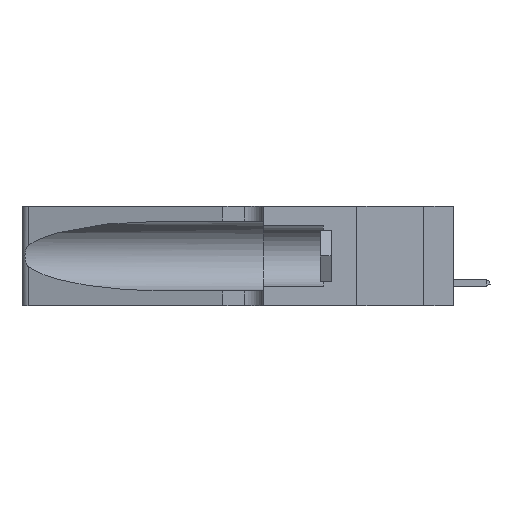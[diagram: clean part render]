
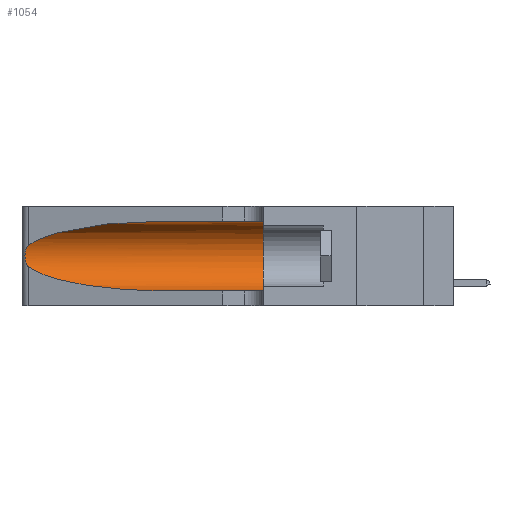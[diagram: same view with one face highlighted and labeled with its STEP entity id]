
A CAD part, left-side view. The second image highlights one B-rep face of the part: STEP entity #1054.
In plain terms, the highlighted cylindrical face has radius 3.308 mm (diameter 6.617 mm), a partial arc.
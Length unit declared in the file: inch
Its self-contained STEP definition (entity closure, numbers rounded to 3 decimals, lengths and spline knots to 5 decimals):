
#74 = ORIENTED_EDGE ( 'NONE', *, *, #16805, .F. ) ;
#197 = VERTEX_POINT ( 'NONE', #497 ) ;
#427 = CARTESIAN_POINT ( 'NONE',  ( 0.1305, 0.72297, 0.31525 ) ) ;
#497 = CARTESIAN_POINT ( 'NONE',  ( 0.1305, 0.72297, 0.31525 ) ) ;
#614 = CARTESIAN_POINT ( 'NONE',  ( 0.25487, 1.22718, 0.22369 ) ) ;
#639 = AXIS2_PLACEMENT_3D ( 'NONE', #3999, #11003, #16444 ) ;
#1054 = ADVANCED_FACE ( 'NONE', ( #14045 ), #2407, .F. ) ;
#1343 = VERTEX_POINT ( 'NONE', #614 ) ;
#1510 = CARTESIAN_POINT ( 'NONE',  ( 0.25487, 1.22718, 0.14631 ) ) ;
#2016 = VECTOR ( 'NONE', #13658, 39.37008 ) ;
#2313 = CARTESIAN_POINT ( 'NONE',  ( 0.25787, 1.23484, 0.2124 ) ) ;
#2407 = CYLINDRICAL_SURFACE ( 'NONE', #639, 0.13025 ) ;
#2548 = CARTESIAN_POINT ( 'NONE',  ( 0.25487, 1.22718, 0.14631 ) ) ;
#2901 = VERTEX_POINT ( 'NONE', #11249 ) ;
#3780 = B_SPLINE_CURVE_WITH_KNOTS ( 'NONE', 3,
 ( #16216, #17584, #7789, #2313, #9340, #13317, #3889, #9224, #8253, #17644, #8194, #9400, #16392, #2548 ),
 .UNSPECIFIED., .F., .F.,
 ( 4, 2, 2, 2, 2, 2, 4 ),
 ( 0., 0.00027, 0.00053, 0.00107, 0.0016, 0.00187, 0.00214 ),
 .UNSPECIFIED. ) ;
#3876 = EDGE_CURVE ( 'NONE', #4979, #2901, #10930, .T. ) ;
#3889 = CARTESIAN_POINT ( 'NONE',  ( 0.26075, 1.23896, 0.19203 ) ) ;
#3999 = CARTESIAN_POINT ( 'NONE',  ( 0.1305, 1.61858, 0.185 ) ) ;
#4387 = CIRCLE ( 'NONE', #9984, 0.13025 ) ;
#4979 = VERTEX_POINT ( 'NONE', #14927 ) ;
#5138 = DIRECTION ( 'NONE',  ( 0., 1., 0. ) ) ;
#5462 = ORIENTED_EDGE ( 'NONE', *, *, #14067, .F. ) ;
#5634 = CARTESIAN_POINT ( 'NONE',  ( 0.1305, 0.72297, 0.05475 ) ) ;
#6020 = ORIENTED_EDGE ( 'NONE', *, *, #17604, .T. ) ;
#6973 = LINE ( 'NONE', #6981, #2016 ) ;
#6981 = CARTESIAN_POINT ( 'NONE',  ( 0.1305, 1.61858, 0.31525 ) ) ;
#7063 = CARTESIAN_POINT ( 'NONE',  ( 0.1305, 1.61858, 0.05475 ) ) ;
#7192 = CARTESIAN_POINT ( 'NONE',  ( 0.25487, 1.22718, 0.22369 ) ) ;
#7325 = EDGE_CURVE ( 'NONE', #1343, #17006, #3780, .T. ) ;
#7789 = CARTESIAN_POINT ( 'NONE',  ( 0.25639, 1.23184, 0.21858 ) ) ;
#8151 = ORIENTED_EDGE ( 'NONE', *, *, #7325, .T. ) ;
#8194 = CARTESIAN_POINT ( 'NONE',  ( 0.25789, 1.23486, 0.15765 ) ) ;
#8253 = CARTESIAN_POINT ( 'NONE',  ( 0.26017, 1.23833, 0.17102 ) ) ;
#8424 = DIRECTION ( 'NONE',  ( 0., -1., 0. ) ) ;
#8612 = CARTESIAN_POINT ( 'NONE',  ( 0.18966, 0.96281, 0.31525 ) ) ;
#9224 = CARTESIAN_POINT ( 'NONE',  ( 0.26075, 1.23896, 0.178 ) ) ;
#9231 = VECTOR ( 'NONE', #8424, 39.37008 ) ;
#9340 = CARTESIAN_POINT ( 'NONE',  ( 0.25854, 1.2359, 0.20912 ) ) ;
#9400 = CARTESIAN_POINT ( 'NONE',  ( 0.25639, 1.23186, 0.15144 ) ) ;
#9636 = EDGE_CURVE ( 'NONE', #17006, #4979, #13362, .T. ) ;
#9984 = AXIS2_PLACEMENT_3D ( 'NONE', #13387, #5138, #15196 ) ;
#10185 = CARTESIAN_POINT ( 'NONE',  ( 0.25487, 1.22718, 0.14631 ) ) ;
#10930 = LINE ( 'NONE', #7063, #9231 ) ;
#11003 = DIRECTION ( 'NONE',  ( 0., -1., 0. ) ) ;
#11182 = CARTESIAN_POINT ( 'NONE',  ( 0.2373, 1.15595, 0.08982 ) ) ;
#11249 = CARTESIAN_POINT ( 'NONE',  ( 0.1305, 0.35, 0.05475 ) ) ;
#13317 = CARTESIAN_POINT ( 'NONE',  ( 0.26018, 1.23835, 0.19895 ) ) ;
#13362 =( BOUNDED_CURVE ( )  B_SPLINE_CURVE ( 3, ( #1510, #11182, #13901, #5634 ),
 .UNSPECIFIED., .F., .T. ) 
 B_SPLINE_CURVE_WITH_KNOTS ( ( 4, 4 ),
 ( 3.44316, 4.71239 ),
 .UNSPECIFIED. ) 
 CURVE ( )  GEOMETRIC_REPRESENTATION_ITEM ( )  RATIONAL_B_SPLINE_CURVE ( ( 1., 0.87, 0.87, 1. ) ) 
 REPRESENTATION_ITEM ( '' )  );
#13387 = CARTESIAN_POINT ( 'NONE',  ( 0.1305, 0.35, 0.185 ) ) ;
#13569 = VERTEX_POINT ( 'NONE', #14386 ) ;
#13658 = DIRECTION ( 'NONE',  ( 0., -1., 0. ) ) ;
#13901 = CARTESIAN_POINT ( 'NONE',  ( 0.18966, 0.96281, 0.05475 ) ) ;
#14045 = FACE_OUTER_BOUND ( 'NONE', #16187, .T. ) ;
#14067 = EDGE_CURVE ( 'NONE', #197, #13569, #6973, .T. ) ;
#14386 = CARTESIAN_POINT ( 'NONE',  ( 0.1305, 0.35, 0.31525 ) ) ;
#14625 = ORIENTED_EDGE ( 'NONE', *, *, #3876, .T. ) ;
#14927 = CARTESIAN_POINT ( 'NONE',  ( 0.1305, 0.72297, 0.05475 ) ) ;
#15196 = DIRECTION ( 'NONE',  ( 0., 0., 1. ) ) ;
#15252 =( BOUNDED_CURVE ( )  B_SPLINE_CURVE ( 3, ( #427, #8612, #15593, #7192 ),
 .UNSPECIFIED., .F., .F. ) 
 B_SPLINE_CURVE_WITH_KNOTS ( ( 4, 4 ),
 ( 1.5708, 2.84003 ),
 .UNSPECIFIED. ) 
 CURVE ( )  GEOMETRIC_REPRESENTATION_ITEM ( )  RATIONAL_B_SPLINE_CURVE ( ( 1., 0.87, 0.87, 1. ) ) 
 REPRESENTATION_ITEM ( '' )  );
#15593 = CARTESIAN_POINT ( 'NONE',  ( 0.2373, 1.15595, 0.28018 ) ) ;
#16187 = EDGE_LOOP ( 'NONE', ( #6020, #8151, #17337, #14625, #74, #5462 ) ) ;
#16216 = CARTESIAN_POINT ( 'NONE',  ( 0.25487, 1.22718, 0.22369 ) ) ;
#16392 = CARTESIAN_POINT ( 'NONE',  ( 0.25555, 1.22993, 0.14849 ) ) ;
#16444 = DIRECTION ( 'NONE',  ( 0., 0., -1. ) ) ;
#16805 = EDGE_CURVE ( 'NONE', #13569, #2901, #4387, .T. ) ;
#17006 = VERTEX_POINT ( 'NONE', #10185 ) ;
#17337 = ORIENTED_EDGE ( 'NONE', *, *, #9636, .T. ) ;
#17584 = CARTESIAN_POINT ( 'NONE',  ( 0.25555, 1.22994, 0.2215 ) ) ;
#17604 = EDGE_CURVE ( 'NONE', #197, #1343, #15252, .T. ) ;
#17644 = CARTESIAN_POINT ( 'NONE',  ( 0.25856, 1.23593, 0.16098 ) ) ;
